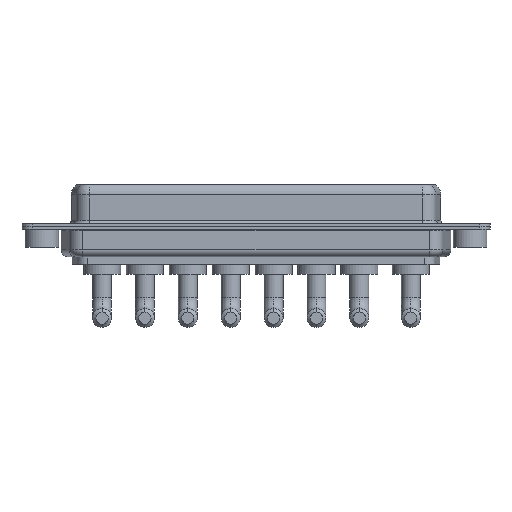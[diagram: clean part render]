
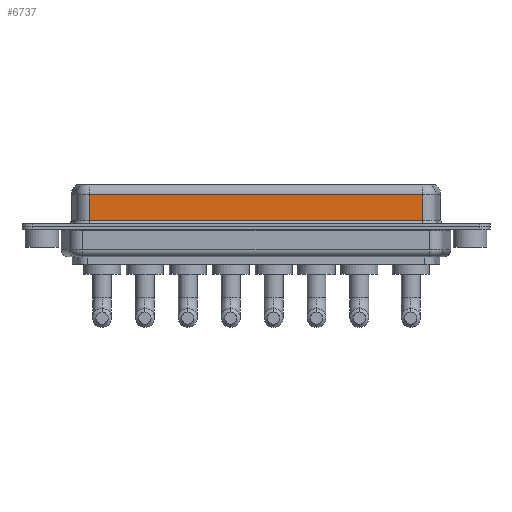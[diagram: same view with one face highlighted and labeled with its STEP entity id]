
A CAD part, front view. The second image highlights one B-rep face of the part: STEP entity #6737.
In plain terms, the highlighted planar face has unit normal (0, -1, 0).
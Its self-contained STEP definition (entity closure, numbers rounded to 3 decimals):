
#41 = CARTESIAN_POINT ( 'NONE',  ( 56.462, -3.95, 4.65 ) ) ;
#60 = LINE ( 'NONE', #4994, #7646 ) ;
#110 = DIRECTION ( 'NONE',  ( -1., 0., 0. ) ) ;
#186 = DIRECTION ( 'NONE',  ( 0., 0., 1. ) ) ;
#483 = CARTESIAN_POINT ( 'NONE',  ( 7.038, -3.95, 0.9 ) ) ;
#582 = VECTOR ( 'NONE', #680, 1000. ) ;
#616 = CARTESIAN_POINT ( 'NONE',  ( 56.462, -3.95, 4.65 ) ) ;
#680 = DIRECTION ( 'NONE',  ( 0., 0., -1. ) ) ;
#1266 = FACE_OUTER_BOUND ( 'NONE', #3865, .T. ) ;
#1680 = ORIENTED_EDGE ( 'NONE', *, *, #10860, .F. ) ;
#1751 = CARTESIAN_POINT ( 'NONE',  ( 7.038, -3.95, 6.4 ) ) ;
#1947 = ORIENTED_EDGE ( 'NONE', *, *, #9297, .T. ) ;
#3154 = LINE ( 'NONE', #11276, #9827 ) ;
#3318 = PLANE ( 'NONE',  #6472 ) ;
#3865 = EDGE_LOOP ( 'NONE', ( #1680, #13259, #1947, #10637 ) ) ;
#4584 = EDGE_CURVE ( 'NONE', #5239, #7481, #3154, .T. ) ;
#4679 = LINE ( 'NONE', #1751, #582 ) ;
#4994 = CARTESIAN_POINT ( 'NONE',  ( 56.462, -3.95, 6.4 ) ) ;
#5239 = VERTEX_POINT ( 'NONE', #483 ) ;
#5545 = VERTEX_POINT ( 'NONE', #11800 ) ;
#6472 = AXIS2_PLACEMENT_3D ( 'NONE', #12401, #7328, #186 ) ;
#6737 = ADVANCED_FACE ( 'NONE', ( #1266 ), #3318, .F. ) ;
#7030 = CARTESIAN_POINT ( 'NONE',  ( 56.462, -3.95, 0.9 ) ) ;
#7328 = DIRECTION ( 'NONE',  ( 0., 1., 0. ) ) ;
#7481 = VERTEX_POINT ( 'NONE', #7030 ) ;
#7646 = VECTOR ( 'NONE', #11903, 1000. ) ;
#7994 = VERTEX_POINT ( 'NONE', #616 ) ;
#8473 = EDGE_CURVE ( 'NONE', #7994, #5545, #12257, .T. ) ;
#9297 = EDGE_CURVE ( 'NONE', #5545, #5239, #4679, .T. ) ;
#9827 = VECTOR ( 'NONE', #10141, 1000. ) ;
#10141 = DIRECTION ( 'NONE',  ( 1., 0., 0. ) ) ;
#10637 = ORIENTED_EDGE ( 'NONE', *, *, #4584, .T. ) ;
#10860 = EDGE_CURVE ( 'NONE', #7994, #7481, #60, .T. ) ;
#11265 = VECTOR ( 'NONE', #110, 1000. ) ;
#11276 = CARTESIAN_POINT ( 'NONE',  ( 56.462, -3.95, 0.9 ) ) ;
#11800 = CARTESIAN_POINT ( 'NONE',  ( 7.038, -3.95, 4.65 ) ) ;
#11903 = DIRECTION ( 'NONE',  ( 0., 0., -1. ) ) ;
#12257 = LINE ( 'NONE', #41, #11265 ) ;
#12401 = CARTESIAN_POINT ( 'NONE',  ( 56.462, -3.95, 6.4 ) ) ;
#13259 = ORIENTED_EDGE ( 'NONE', *, *, #8473, .T. ) ;
